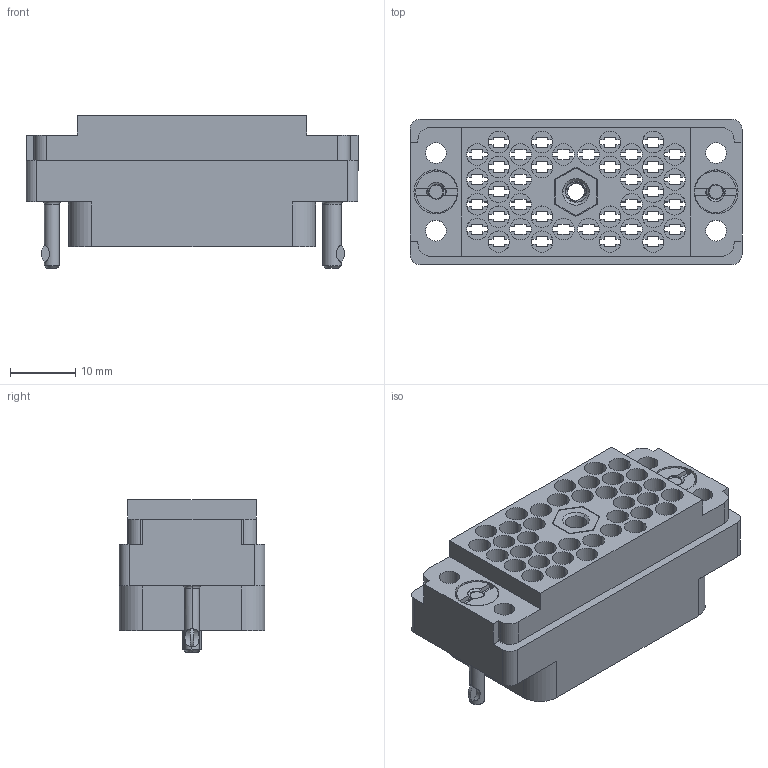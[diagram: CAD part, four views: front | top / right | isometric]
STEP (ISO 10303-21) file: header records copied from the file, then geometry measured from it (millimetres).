
FILE_DESCRIPTION (( 'STEP AP203' ), '1' );
FILE_NAME ('516-038-000-502.STEP', '2020-03-09T18:40:36', ( '' ), ( '' ), 'SwSTEP 2.0', 'SolidWorks 2016', '' );
FILE_SCHEMA (( 'CONFIG_CONTROL_DESIGN' ));
Length unit declared in the file: inch
Products named in the file (6): 516 Plug Insulator_038; 516-222-038-102_038; 516-252-021-102_038; 516-222-038-102_039; 516-252-035-100_516-252-035-100; 516-038-000-502
Assembly tree (6 placements, depth 2):
  516-038-000-502
    516 Plug Insulator_038
    516-252-021-102_038  x2
    516-222-038-102_038
    516-252-035-100_516-252-035-100
    516-222-038-102_039
Bounding box: 50.8 x 22.25 x 23.37 mm (x, y, z)
Volume: 9257 mm3; surface area: 12616.9 mm2
Topology: 6 solids, 6 shells, 1123 faces, 3204 edges, 2116 vertices
Faces by surface type: plane 696, cylinder 335, cone 46, bspline 42, torus 4
Entity records: 42943 total; most frequent: CARTESIAN_POINT 13518, ORIENTED_EDGE 6228, DIRECTION 5810, EDGE_CURVE 3114, LINE 2104, VECTOR 2104, VERTEX_POINT 2056, AXIS2_PLACEMENT_3D 1853
